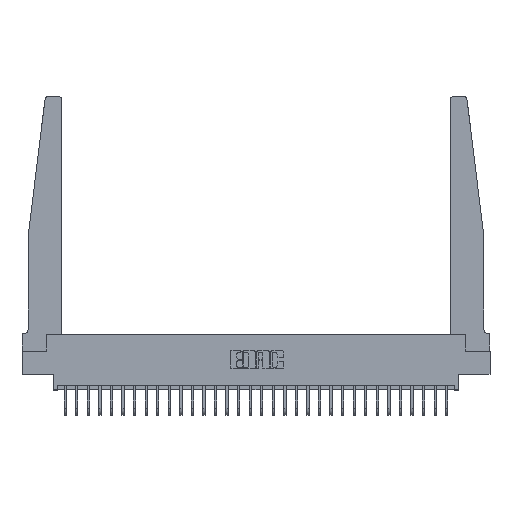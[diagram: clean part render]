
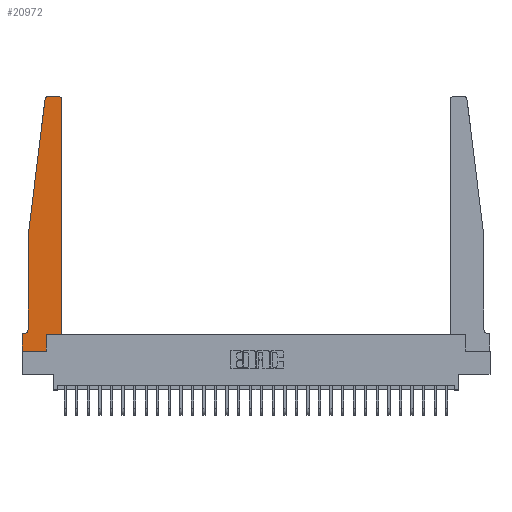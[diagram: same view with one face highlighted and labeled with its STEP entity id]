
A CAD part, top view. The second image highlights one B-rep face of the part: STEP entity #20972.
In plain terms, the highlighted planar face has unit normal (0, 0, 1).
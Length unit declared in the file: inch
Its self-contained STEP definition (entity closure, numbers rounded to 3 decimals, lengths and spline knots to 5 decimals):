
#348 = CARTESIAN_POINT ( 'NONE',  ( 0.24675, 2.72367, 0.37 ) ) ;
#383 = CARTESIAN_POINT ( 'NONE',  ( 0.2605, 0.18, 0.37 ) ) ;
#427 = ORIENTED_EDGE ( 'NONE', *, *, #8782, .T. ) ;
#536 = DIRECTION ( 'NONE',  ( 0., 1., 0. ) ) ;
#602 = DIRECTION ( 'NONE',  ( 0., 1., 0. ) ) ;
#686 = CARTESIAN_POINT ( 'NONE',  ( 0.065, 1.25, 0.37 ) ) ;
#988 = VERTEX_POINT ( 'NONE', #348 ) ;
#1524 = CARTESIAN_POINT ( 'NONE',  ( 0., 0., 0.37 ) ) ;
#2315 = DIRECTION ( 'NONE',  ( 0., 0., 1. ) ) ;
#3024 = EDGE_CURVE ( 'NONE', #13651, #24069, #4075, .T. ) ;
#3134 = ORIENTED_EDGE ( 'NONE', *, *, #8284, .T. ) ;
#3281 = CARTESIAN_POINT ( 'NONE',  ( 0.25, 2.75, 0.37 ) ) ;
#3299 = EDGE_CURVE ( 'NONE', #988, #24862, #16823, .T. ) ;
#3606 = CIRCLE ( 'NONE', #20881, 0.03 ) ;
#3817 = LINE ( 'NONE', #1524, #26497 ) ;
#4075 = LINE ( 'NONE', #29344, #5200 ) ;
#4344 = ORIENTED_EDGE ( 'NONE', *, *, #19157, .T. ) ;
#4826 = VECTOR ( 'NONE', #602, 39.37008 ) ;
#4990 = CARTESIAN_POINT ( 'NONE',  ( 0.065, 1.25, 0.37 ) ) ;
#5200 = VECTOR ( 'NONE', #10851, 39.37008 ) ;
#5633 = VECTOR ( 'NONE', #15348, 39.37008 ) ;
#6463 = EDGE_CURVE ( 'NONE', #24862, #19327, #7617, .T. ) ;
#6948 = FACE_OUTER_BOUND ( 'NONE', #24725, .T. ) ;
#7119 = ORIENTED_EDGE ( 'NONE', *, *, #17255, .T. ) ;
#7374 = ORIENTED_EDGE ( 'NONE', *, *, #3024, .T. ) ;
#7617 = LINE ( 'NONE', #686, #13035 ) ;
#7767 = EDGE_CURVE ( 'NONE', #13784, #988, #3606, .T. ) ;
#8247 = LINE ( 'NONE', #20164, #24728 ) ;
#8284 = EDGE_CURVE ( 'NONE', #19327, #16676, #16450, .T. ) ;
#8782 = EDGE_CURVE ( 'NONE', #16676, #25166, #20644, .T. ) ;
#9123 = ORIENTED_EDGE ( 'NONE', *, *, #3299, .T. ) ;
#9394 = CARTESIAN_POINT ( 'NONE',  ( 0., 0.1875, 0.37 ) ) ;
#9414 = CARTESIAN_POINT ( 'NONE',  ( 0.425, 0.18, 0.37 ) ) ;
#9516 = CARTESIAN_POINT ( 'NONE',  ( 0.425, 0.18, 0.37 ) ) ;
#9755 = LINE ( 'NONE', #383, #10002 ) ;
#10002 = VECTOR ( 'NONE', #536, 39.37008 ) ;
#10154 = VERTEX_POINT ( 'NONE', #19769 ) ;
#10399 = DIRECTION ( 'NONE',  ( 1., 0., 0. ) ) ;
#10671 = CARTESIAN_POINT ( 'NONE',  ( 0.065, 0.2375, 0.37 ) ) ;
#10851 = DIRECTION ( 'NONE',  ( 1., 0., 0. ) ) ;
#11124 = CARTESIAN_POINT ( 'NONE',  ( 0.2605, 0., 0.37 ) ) ;
#11554 = CARTESIAN_POINT ( 'NONE',  ( 0.015, 0.1875, 0.37 ) ) ;
#11897 = CARTESIAN_POINT ( 'NONE',  ( 0.015, 0.2375, 0.37 ) ) ;
#12056 = CARTESIAN_POINT ( 'NONE',  ( 0.065, 1.25, 0.37 ) ) ;
#12074 = DIRECTION ( 'NONE',  ( 0., -1., 0. ) ) ;
#12252 = CARTESIAN_POINT ( 'NONE',  ( 0.395, 2.72, 0.37 ) ) ;
#12699 = DIRECTION ( 'NONE',  ( -1., 0., 0. ) ) ;
#12740 = ORIENTED_EDGE ( 'NONE', *, *, #15556, .T. ) ;
#12802 = ORIENTED_EDGE ( 'NONE', *, *, #6463, .T. ) ;
#13035 = VECTOR ( 'NONE', #12074, 39.37008 ) ;
#13461 = CARTESIAN_POINT ( 'NONE',  ( 0.2605, 0.18, 0.37 ) ) ;
#13651 = VERTEX_POINT ( 'NONE', #13461 ) ;
#13784 = VERTEX_POINT ( 'NONE', #28070 ) ;
#14324 = VERTEX_POINT ( 'NONE', #24459 ) ;
#14370 = DIRECTION ( 'NONE',  ( -0.122, -0.992, 0. ) ) ;
#14576 = EDGE_CURVE ( 'NONE', #14903, #13651, #9755, .T. ) ;
#14903 = VERTEX_POINT ( 'NONE', #11124 ) ;
#15013 = DIRECTION ( 'NONE',  ( 0., 0., 1. ) ) ;
#15348 = DIRECTION ( 'NONE',  ( -1., 0., 0. ) ) ;
#15556 = EDGE_CURVE ( 'NONE', #21965, #14903, #8247, .T. ) ;
#16010 = VECTOR ( 'NONE', #14370, 39.37008 ) ;
#16082 = AXIS2_PLACEMENT_3D ( 'NONE', #12252, #22169, #19703 ) ;
#16450 = CIRCLE ( 'NONE', #27756, 0.05 ) ;
#16615 = LINE ( 'NONE', #9516, #4826 ) ;
#16676 = VERTEX_POINT ( 'NONE', #11554 ) ;
#16823 = LINE ( 'NONE', #12056, #16010 ) ;
#17255 = EDGE_CURVE ( 'NONE', #14324, #10154, #23500, .T. ) ;
#19050 = CARTESIAN_POINT ( 'NONE',  ( 0.27653, 2.72, 0.37 ) ) ;
#19157 = EDGE_CURVE ( 'NONE', #10154, #13784, #24413, .T. ) ;
#19327 = VERTEX_POINT ( 'NONE', #10671 ) ;
#19703 = DIRECTION ( 'NONE',  ( 1., 0., 0. ) ) ;
#19769 = CARTESIAN_POINT ( 'NONE',  ( 0.395, 2.75, 0.37 ) ) ;
#20164 = CARTESIAN_POINT ( 'NONE',  ( 0., 0., 0.37 ) ) ;
#20358 = DIRECTION ( 'NONE',  ( 0., -1., 0. ) ) ;
#20644 = LINE ( 'NONE', #27667, #5633 ) ;
#20881 = AXIS2_PLACEMENT_3D ( 'NONE', #19050, #15013, #24129 ) ;
#20972 = ADVANCED_FACE ( 'NONE', ( #6948 ), #21029, .T. ) ;
#21029 = PLANE ( 'NONE',  #23167 ) ;
#21055 = CARTESIAN_POINT ( 'NONE',  ( 0., 0.1875, 0.37 ) ) ;
#21343 = DIRECTION ( 'NONE',  ( 0., 0., -1. ) ) ;
#21965 = VERTEX_POINT ( 'NONE', #28547 ) ;
#22169 = DIRECTION ( 'NONE',  ( 0., 0., 1. ) ) ;
#22636 = ORIENTED_EDGE ( 'NONE', *, *, #27138, .T. ) ;
#23068 = ORIENTED_EDGE ( 'NONE', *, *, #14576, .T. ) ;
#23167 = AXIS2_PLACEMENT_3D ( 'NONE', #9394, #2315, #28320 ) ;
#23500 = CIRCLE ( 'NONE', #16082, 0.03 ) ;
#24069 = VERTEX_POINT ( 'NONE', #9414 ) ;
#24129 = DIRECTION ( 'NONE',  ( 1., 0., 0. ) ) ;
#24178 = ORIENTED_EDGE ( 'NONE', *, *, #28098, .T. ) ;
#24243 = ORIENTED_EDGE ( 'NONE', *, *, #7767, .T. ) ;
#24413 = LINE ( 'NONE', #3281, #25523 ) ;
#24459 = CARTESIAN_POINT ( 'NONE',  ( 0.425, 2.72, 0.37 ) ) ;
#24725 = EDGE_LOOP ( 'NONE', ( #4344, #24243, #9123, #12802, #3134, #427, #22636, #12740, #23068, #7374, #24178, #7119 ) ) ;
#24728 = VECTOR ( 'NONE', #10399, 39.37008 ) ;
#24862 = VERTEX_POINT ( 'NONE', #4990 ) ;
#25166 = VERTEX_POINT ( 'NONE', #21055 ) ;
#25523 = VECTOR ( 'NONE', #12699, 39.37008 ) ;
#26084 = DIRECTION ( 'NONE',  ( -1., 0., 0. ) ) ;
#26497 = VECTOR ( 'NONE', #20358, 39.37008 ) ;
#27138 = EDGE_CURVE ( 'NONE', #25166, #21965, #3817, .T. ) ;
#27667 = CARTESIAN_POINT ( 'NONE',  ( 0.065, 0.1875, 0.37 ) ) ;
#27756 = AXIS2_PLACEMENT_3D ( 'NONE', #11897, #21343, #26084 ) ;
#28070 = CARTESIAN_POINT ( 'NONE',  ( 0.27653, 2.75, 0.37 ) ) ;
#28098 = EDGE_CURVE ( 'NONE', #24069, #14324, #16615, .T. ) ;
#28320 = DIRECTION ( 'NONE',  ( 1., 0., 0. ) ) ;
#28547 = CARTESIAN_POINT ( 'NONE',  ( 0., 0., 0.37 ) ) ;
#29344 = CARTESIAN_POINT ( 'NONE',  ( 0.425, 0.18, 0.37 ) ) ;
